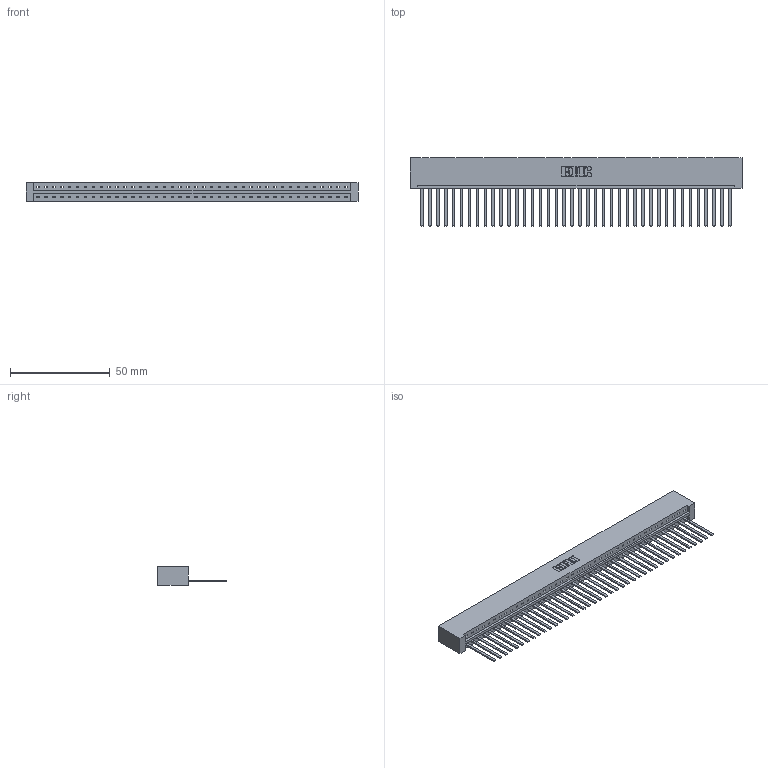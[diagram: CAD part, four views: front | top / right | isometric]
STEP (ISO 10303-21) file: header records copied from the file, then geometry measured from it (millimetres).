
FILE_DESCRIPTION (( 'STEP AP203' ), '1' );
FILE_NAME ('333-040-544-101.STEP', '2018-08-03T14:25:47', ( '' ), ( '' ), 'SwSTEP 2.0', 'SolidWorks 2016', '' );
FILE_SCHEMA (( 'CONFIG_CONTROL_DESIGN' ));
Length unit declared in the file: inch
Products named in the file (3): 333-040-544-101; 333 Part_Lugless; 345-292-001_345-293-144
Assembly tree (41 placements, depth 2):
  333-040-544-101
    333 Part_Lugless
    345-292-001_345-293-144  x40
Bounding box: 166.75 x 34.3 x 9.4 mm (x, y, z)
Volume: 17838.7 mm3; surface area: 20750.9 mm2
Topology: 41 solids, 41 shells, 2186 faces, 6607 edges, 4350 vertices
Faces by surface type: plane 1586, cylinder 600
Entity records: 24251 total; most frequent: CARTESIAN_POINT 4190, ORIENTED_EDGE 4166, DIRECTION 3527, EDGE_CURVE 2083, LINE 1967, VECTOR 1967, VERTEX_POINT 1386, AXIS2_PLACEMENT_3D 780
